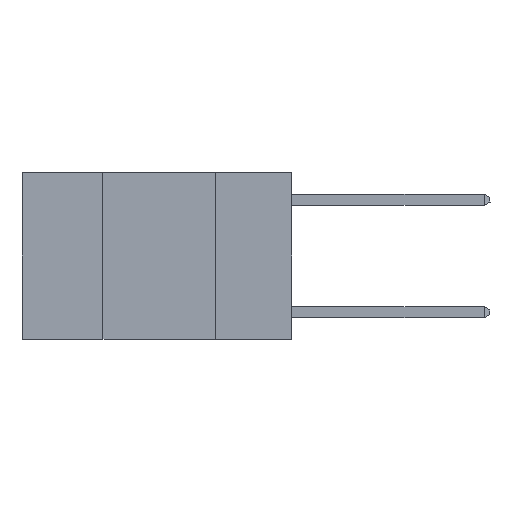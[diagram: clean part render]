
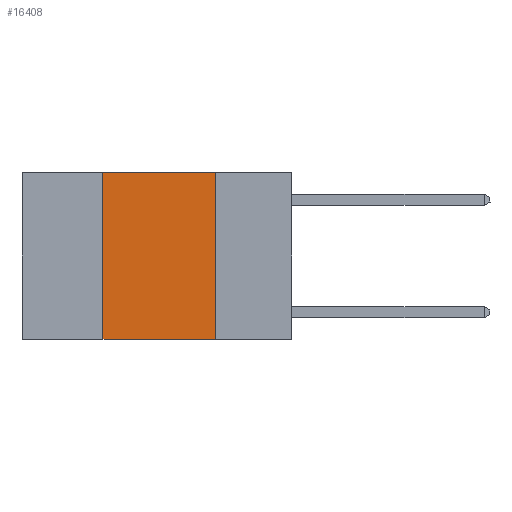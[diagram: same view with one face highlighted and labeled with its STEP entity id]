
A CAD part, left-side view. The second image highlights one B-rep face of the part: STEP entity #16408.
In plain terms, the highlighted planar face has unit normal (-1, 0, 0).
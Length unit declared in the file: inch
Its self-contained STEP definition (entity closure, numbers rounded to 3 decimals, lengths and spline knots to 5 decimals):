
#705 = EDGE_CURVE ( 'NONE', #20223, #16009, #27849, .T. ) ;
#1358 = DIRECTION ( 'NONE',  ( 0., 0., 1. ) ) ;
#1677 = DIRECTION ( 'NONE',  ( 1., 0., 0. ) ) ;
#2538 = CARTESIAN_POINT ( 'NONE',  ( 0., 0.42, -0.37 ) ) ;
#2790 = EDGE_CURVE ( 'NONE', #14490, #20223, #8894, .T. ) ;
#4563 = DIRECTION ( 'NONE',  ( 0., -1., 0. ) ) ;
#5867 = CARTESIAN_POINT ( 'NONE',  ( 0., 0.17, -0.37 ) ) ;
#6359 = DIRECTION ( 'NONE',  ( 0., 0., -1. ) ) ;
#6470 = CARTESIAN_POINT ( 'NONE',  ( 0., 0.6, 0. ) ) ;
#8894 = LINE ( 'NONE', #24734, #26634 ) ;
#8901 = PLANE ( 'NONE',  #27376 ) ;
#10639 = CARTESIAN_POINT ( 'NONE',  ( 0., 0.6, 0. ) ) ;
#11245 = ORIENTED_EDGE ( 'NONE', *, *, #13675, .T. ) ;
#11247 = DIRECTION ( 'NONE',  ( 0., 0., -1. ) ) ;
#11406 = ORIENTED_EDGE ( 'NONE', *, *, #705, .F. ) ;
#11811 = CARTESIAN_POINT ( 'NONE',  ( 0., 0.17, 0. ) ) ;
#11967 = LINE ( 'NONE', #22715, #28888 ) ;
#12612 = ORIENTED_EDGE ( 'NONE', *, *, #2790, .F. ) ;
#13675 = EDGE_CURVE ( 'NONE', #14490, #18940, #15813, .T. ) ;
#14490 = VERTEX_POINT ( 'NONE', #2538 ) ;
#15813 = LINE ( 'NONE', #16262, #16562 ) ;
#16009 = VERTEX_POINT ( 'NONE', #11811 ) ;
#16262 = CARTESIAN_POINT ( 'NONE',  ( 0., 0.6, -0.37 ) ) ;
#16408 = ADVANCED_FACE ( 'NONE', ( #17503 ), #8901, .F. ) ;
#16562 = VECTOR ( 'NONE', #4563, 39.37008 ) ;
#17039 = EDGE_LOOP ( 'NONE', ( #17454, #11406, #12612, #11245 ) ) ;
#17454 = ORIENTED_EDGE ( 'NONE', *, *, #19583, .F. ) ;
#17503 = FACE_OUTER_BOUND ( 'NONE', #17039, .T. ) ;
#18940 = VERTEX_POINT ( 'NONE', #5867 ) ;
#19583 = EDGE_CURVE ( 'NONE', #16009, #18940, #11967, .T. ) ;
#20223 = VERTEX_POINT ( 'NONE', #20390 ) ;
#20390 = CARTESIAN_POINT ( 'NONE',  ( 0., 0.42, 0. ) ) ;
#21091 = VECTOR ( 'NONE', #29000, 39.37008 ) ;
#22715 = CARTESIAN_POINT ( 'NONE',  ( 0., 0.17, 0. ) ) ;
#24734 = CARTESIAN_POINT ( 'NONE',  ( 0., 0.42, 0. ) ) ;
#26634 = VECTOR ( 'NONE', #1358, 39.37008 ) ;
#27376 = AXIS2_PLACEMENT_3D ( 'NONE', #6470, #1677, #11247 ) ;
#27849 = LINE ( 'NONE', #10639, #21091 ) ;
#28888 = VECTOR ( 'NONE', #6359, 39.37008 ) ;
#29000 = DIRECTION ( 'NONE',  ( 0., -1., 0. ) ) ;
